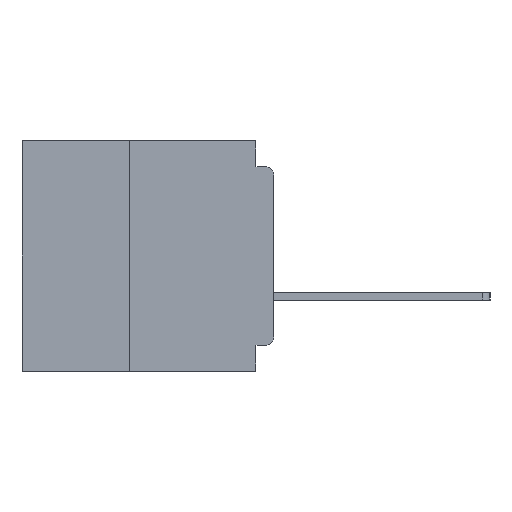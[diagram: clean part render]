
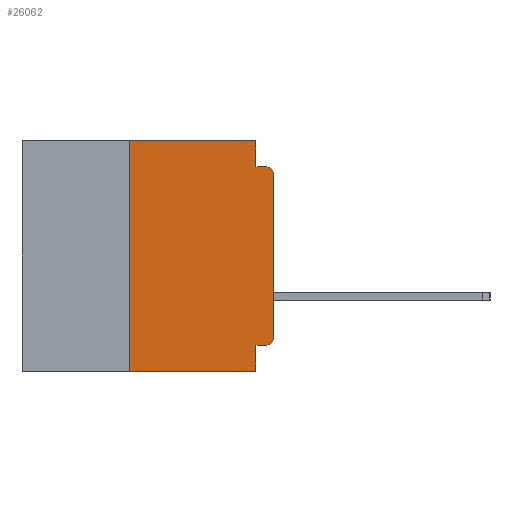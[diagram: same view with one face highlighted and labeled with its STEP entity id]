
A CAD part, left-side view. The second image highlights one B-rep face of the part: STEP entity #26062.
In plain terms, the highlighted planar face has unit normal (-1, 0, 0).
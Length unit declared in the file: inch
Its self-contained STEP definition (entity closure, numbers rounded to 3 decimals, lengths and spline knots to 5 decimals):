
#668 = VERTEX_POINT ( 'NONE', #6260 ) ;
#897 = VECTOR ( 'NONE', #16279, 39.37008 ) ;
#1162 = ORIENTED_EDGE ( 'NONE', *, *, #17093, .T. ) ;
#1417 = CARTESIAN_POINT ( 'NONE',  ( 0., 0., -0.34 ) ) ;
#1641 = CARTESIAN_POINT ( 'NONE',  ( 0., 0.015, -0.355 ) ) ;
#1932 = CARTESIAN_POINT ( 'NONE',  ( 0., 0., -0.06 ) ) ;
#1971 = LINE ( 'NONE', #26363, #897 ) ;
#2009 = AXIS2_PLACEMENT_3D ( 'NONE', #19699, #43033, #23044 ) ;
#2278 = EDGE_CURVE ( 'NONE', #33355, #31879, #1971, .T. ) ;
#2919 = EDGE_CURVE ( 'NONE', #11232, #18010, #18133, .T. ) ;
#4789 = DIRECTION ( 'NONE',  ( 0., -1., 0. ) ) ;
#4903 = VERTEX_POINT ( 'NONE', #11358 ) ;
#4959 = AXIS2_PLACEMENT_3D ( 'NONE', #16151, #39517, #19520 ) ;
#5360 = LINE ( 'NONE', #33288, #39873 ) ;
#5425 = LINE ( 'NONE', #16633, #22181 ) ;
#6143 = CIRCLE ( 'NONE', #32936, 0.015 ) ;
#6199 = EDGE_CURVE ( 'NONE', #31879, #13292, #6143, .T. ) ;
#6260 = CARTESIAN_POINT ( 'NONE',  ( 0., 0.25, 0. ) ) ;
#7313 = CARTESIAN_POINT ( 'NONE',  ( 0., 0., -0.045 ) ) ;
#7353 = EDGE_LOOP ( 'NONE', ( #34156, #11173, #38544, #24734, #28341, #10628, #1162, #17054, #34739, #8340 ) ) ;
#8340 = ORIENTED_EDGE ( 'NONE', *, *, #31511, .T. ) ;
#9366 = CARTESIAN_POINT ( 'NONE',  ( 0., 0.031, -0.4 ) ) ;
#10628 = ORIENTED_EDGE ( 'NONE', *, *, #43297, .F. ) ;
#11173 = ORIENTED_EDGE ( 'NONE', *, *, #6199, .T. ) ;
#11232 = VERTEX_POINT ( 'NONE', #40893 ) ;
#11358 = CARTESIAN_POINT ( 'NONE',  ( 0., 0.031, -0.355 ) ) ;
#11360 = CARTESIAN_POINT ( 'NONE',  ( 0., 0.437, 0. ) ) ;
#12317 = DIRECTION ( 'NONE',  ( 0., 0., -1. ) ) ;
#13265 = DIRECTION ( 'NONE',  ( 0., 1., 0. ) ) ;
#13292 = VERTEX_POINT ( 'NONE', #15428 ) ;
#14658 = CARTESIAN_POINT ( 'NONE',  ( 0., 0.25, -0.4 ) ) ;
#14677 = VECTOR ( 'NONE', #12317, 39.37008 ) ;
#15428 = CARTESIAN_POINT ( 'NONE',  ( 0., 0.015, -0.045 ) ) ;
#15677 = DIRECTION ( 'NONE',  ( -1., 0., 0. ) ) ;
#15728 = LINE ( 'NONE', #22294, #14677 ) ;
#16151 = CARTESIAN_POINT ( 'NONE',  ( 0., 0.015, -0.34 ) ) ;
#16279 = DIRECTION ( 'NONE',  ( 0., 0., 1. ) ) ;
#16633 = CARTESIAN_POINT ( 'NONE',  ( 0., 0.25, -0.4 ) ) ;
#17054 = ORIENTED_EDGE ( 'NONE', *, *, #24073, .F. ) ;
#17093 = EDGE_CURVE ( 'NONE', #38083, #42569, #5360, .T. ) ;
#17096 = VECTOR ( 'NONE', #26594, 39.37008 ) ;
#17846 = VECTOR ( 'NONE', #13265, 39.37008 ) ;
#18010 = VERTEX_POINT ( 'NONE', #18921 ) ;
#18133 = LINE ( 'NONE', #33290, #17096 ) ;
#18739 = CIRCLE ( 'NONE', #4959, 0.015 ) ;
#18921 = CARTESIAN_POINT ( 'NONE',  ( 0., 0.031, -0.045 ) ) ;
#19520 = DIRECTION ( 'NONE',  ( 0., 0., -1. ) ) ;
#19699 = CARTESIAN_POINT ( 'NONE',  ( 0., 0.437, 0. ) ) ;
#22181 = VECTOR ( 'NONE', #43324, 39.37008 ) ;
#22294 = CARTESIAN_POINT ( 'NONE',  ( 0., 0.031, -0.4 ) ) ;
#22860 = VECTOR ( 'NONE', #27342, 39.37008 ) ;
#23044 = DIRECTION ( 'NONE',  ( 0., 0., -1. ) ) ;
#23904 = LINE ( 'NONE', #7313, #22860 ) ;
#24073 = EDGE_CURVE ( 'NONE', #4903, #42569, #15728, .T. ) ;
#24734 = ORIENTED_EDGE ( 'NONE', *, *, #2919, .F. ) ;
#25670 = LINE ( 'NONE', #33274, #17846 ) ;
#26062 = ADVANCED_FACE ( 'NONE', ( #32316 ), #32952, .F. ) ;
#26363 = CARTESIAN_POINT ( 'NONE',  ( 0., 0., 0. ) ) ;
#26594 = DIRECTION ( 'NONE',  ( 0., 0., -1. ) ) ;
#27342 = DIRECTION ( 'NONE',  ( 0., -1., 0. ) ) ;
#28341 = ORIENTED_EDGE ( 'NONE', *, *, #41226, .F. ) ;
#29172 = VECTOR ( 'NONE', #4789, 39.37008 ) ;
#29883 = EDGE_CURVE ( 'NONE', #36295, #4903, #25670, .T. ) ;
#30206 = LINE ( 'NONE', #11360, #29172 ) ;
#31511 = EDGE_CURVE ( 'NONE', #36295, #33355, #18739, .T. ) ;
#31879 = VERTEX_POINT ( 'NONE', #1932 ) ;
#32298 = EDGE_CURVE ( 'NONE', #18010, #13292, #23904, .T. ) ;
#32316 = FACE_OUTER_BOUND ( 'NONE', #7353, .T. ) ;
#32936 = AXIS2_PLACEMENT_3D ( 'NONE', #35658, #15677, #39035 ) ;
#32952 = PLANE ( 'NONE',  #2009 ) ;
#33274 = CARTESIAN_POINT ( 'NONE',  ( 0., 0., -0.355 ) ) ;
#33288 = CARTESIAN_POINT ( 'NONE',  ( 0., 0.437, -0.4 ) ) ;
#33290 = CARTESIAN_POINT ( 'NONE',  ( 0., 0.031, 0. ) ) ;
#33355 = VERTEX_POINT ( 'NONE', #1417 ) ;
#34156 = ORIENTED_EDGE ( 'NONE', *, *, #2278, .T. ) ;
#34739 = ORIENTED_EDGE ( 'NONE', *, *, #29883, .F. ) ;
#35658 = CARTESIAN_POINT ( 'NONE',  ( 0., 0.015, -0.06 ) ) ;
#36295 = VERTEX_POINT ( 'NONE', #1641 ) ;
#38083 = VERTEX_POINT ( 'NONE', #14658 ) ;
#38544 = ORIENTED_EDGE ( 'NONE', *, *, #32298, .F. ) ;
#39035 = DIRECTION ( 'NONE',  ( 0., 0., -1. ) ) ;
#39517 = DIRECTION ( 'NONE',  ( -1., 0., 0. ) ) ;
#39873 = VECTOR ( 'NONE', #43357, 39.37008 ) ;
#40893 = CARTESIAN_POINT ( 'NONE',  ( 0., 0.031, 0. ) ) ;
#41226 = EDGE_CURVE ( 'NONE', #668, #11232, #30206, .T. ) ;
#42569 = VERTEX_POINT ( 'NONE', #9366 ) ;
#43033 = DIRECTION ( 'NONE',  ( 1., 0., 0. ) ) ;
#43297 = EDGE_CURVE ( 'NONE', #38083, #668, #5425, .T. ) ;
#43324 = DIRECTION ( 'NONE',  ( 0., 0., 1. ) ) ;
#43357 = DIRECTION ( 'NONE',  ( 0., -1., 0. ) ) ;
